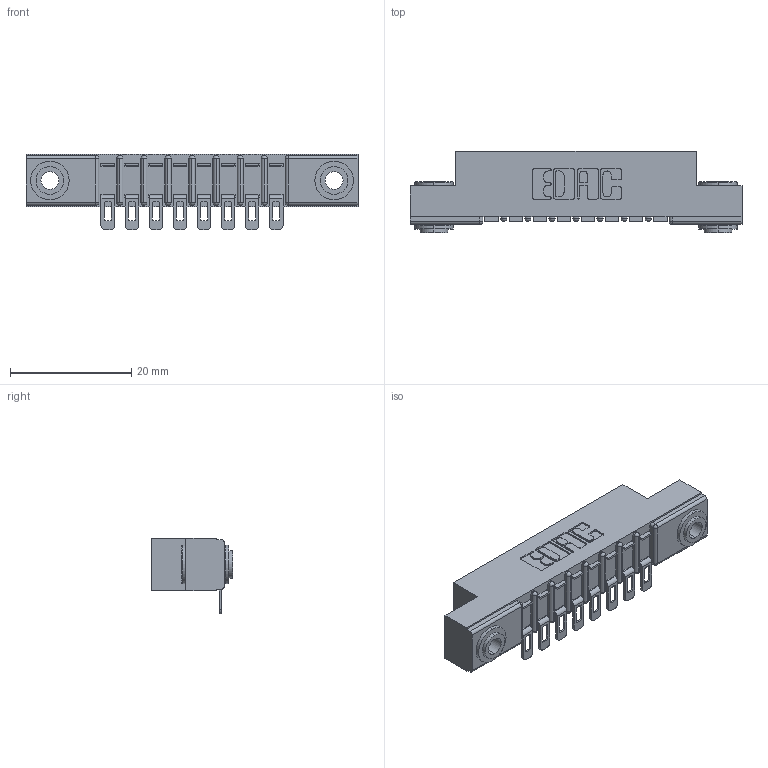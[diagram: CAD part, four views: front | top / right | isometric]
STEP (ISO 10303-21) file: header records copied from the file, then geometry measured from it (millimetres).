
FILE_DESCRIPTION (( 'STEP AP203' ), '1' );
FILE_NAME ('307-008-554-103.STEP', '2019-09-04T18:34:41', ( '' ), ( '' ), 'SwSTEP 2.0', 'SolidWorks 2016', '' );
FILE_SCHEMA (( 'CONFIG_CONTROL_DESIGN' ));
Length unit declared in the file: inch
Products named in the file (4): 307-290-002_554; 307 Part_.156 Dia Mounting Holes; 345-250-002_345-250-002-102; 307-008-554-103
Assembly tree (11 placements, depth 2):
  307-008-554-103
    307 Part_.156 Dia Mounting Holes
    307-290-002_554  x8
    345-250-002_345-250-002-102  x2
Bounding box: 54.71 x 13.36 x 12.52 mm (x, y, z)
Volume: 3608.8 mm3; surface area: 6062.2 mm2
Topology: 11 solids, 11 shells, 827 faces, 2459 edges, 1610 vertices
Faces by surface type: plane 462, cylinder 339, sphere 18, cone 8
Entity records: 13080 total; most frequent: CARTESIAN_POINT 2179, ORIENTED_EDGE 2160, DIRECTION 2154, EDGE_CURVE 1080, VECTOR 796, LINE 796, VERTEX_POINT 704, AXIS2_PLACEMENT_3D 679
